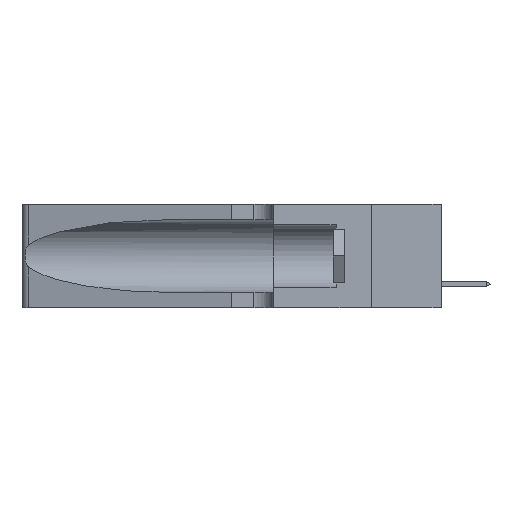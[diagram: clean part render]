
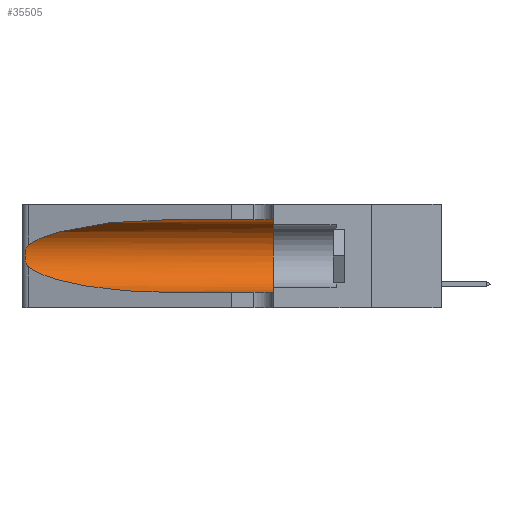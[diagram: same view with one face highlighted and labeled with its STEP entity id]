
A CAD part, left-side view. The second image highlights one B-rep face of the part: STEP entity #35505.
In plain terms, the highlighted cylindrical face has radius 3.308 mm (diameter 6.617 mm), a partial arc.
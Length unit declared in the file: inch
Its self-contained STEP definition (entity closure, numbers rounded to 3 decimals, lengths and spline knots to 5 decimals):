
#619 = CARTESIAN_POINT ( 'NONE',  ( 0.1305, 1.61858, 0.185 ) ) ;
#725 = DIRECTION ( 'NONE',  ( 0., -1., 0. ) ) ;
#741 = EDGE_CURVE ( 'NONE', #9641, #40267, #35137, .T. ) ;
#1351 = CARTESIAN_POINT ( 'NONE',  ( 0.25487, 1.22718, 0.14631 ) ) ;
#1749 = VERTEX_POINT ( 'NONE', #32545 ) ;
#2171 = CARTESIAN_POINT ( 'NONE',  ( 0.18966, 0.96281, 0.31525 ) ) ;
#2450 =( BOUNDED_CURVE ( )  B_SPLINE_CURVE ( 3, ( #1351, #26617, #44153, #33369 ),
 .UNSPECIFIED., .F., .T. ) 
 B_SPLINE_CURVE_WITH_KNOTS ( ( 4, 4 ),
 ( 3.44316, 4.71239 ),
 .UNSPECIFIED. ) 
 CURVE ( )  GEOMETRIC_REPRESENTATION_ITEM ( )  RATIONAL_B_SPLINE_CURVE ( ( 1., 0.87, 0.87, 1. ) ) 
 REPRESENTATION_ITEM ( '' )  );
#2625 = EDGE_CURVE ( 'NONE', #21936, #18528, #22553, .T. ) ;
#3529 = ORIENTED_EDGE ( 'NONE', *, *, #741, .T. ) ;
#3976 = CARTESIAN_POINT ( 'NONE',  ( 0.25787, 1.23484, 0.2124 ) ) ;
#4115 = DIRECTION ( 'NONE',  ( 0., 0., -1. ) ) ;
#6848 = EDGE_CURVE ( 'NONE', #1749, #18528, #18151, .T. ) ;
#7221 = CARTESIAN_POINT ( 'NONE',  ( 0.1305, 1.61858, 0.31525 ) ) ;
#7263 = LINE ( 'NONE', #7221, #25414 ) ;
#7407 = CARTESIAN_POINT ( 'NONE',  ( 0.26018, 1.23835, 0.19895 ) ) ;
#7546 = CARTESIAN_POINT ( 'NONE',  ( 0.26017, 1.23833, 0.17102 ) ) ;
#8415 = CARTESIAN_POINT ( 'NONE',  ( 0.1305, 0.72297, 0.05475 ) ) ;
#9257 = CARTESIAN_POINT ( 'NONE',  ( 0.25487, 1.22718, 0.22369 ) ) ;
#9641 = VERTEX_POINT ( 'NONE', #41501 ) ;
#10827 = CARTESIAN_POINT ( 'NONE',  ( 0.26075, 1.23896, 0.19203 ) ) ;
#10860 = DIRECTION ( 'NONE',  ( 0., 0., 1. ) ) ;
#12087 = VECTOR ( 'NONE', #15900, 39.37008 ) ;
#13704 = EDGE_LOOP ( 'NONE', ( #34426, #3529, #33341, #21244, #24357, #30673 ) ) ;
#14354 = CARTESIAN_POINT ( 'NONE',  ( 0.26075, 1.23896, 0.178 ) ) ;
#14659 = CARTESIAN_POINT ( 'NONE',  ( 0.25555, 1.22993, 0.14849 ) ) ;
#15741 = CARTESIAN_POINT ( 'NONE',  ( 0.1305, 1.61858, 0.05475 ) ) ;
#15900 = DIRECTION ( 'NONE',  ( 0., -1., 0. ) ) ;
#16974 = CARTESIAN_POINT ( 'NONE',  ( 0.25487, 1.22718, 0.14631 ) ) ;
#16994 = FACE_OUTER_BOUND ( 'NONE', #13704, .T. ) ;
#18151 = CIRCLE ( 'NONE', #33225, 0.13025 ) ;
#18528 = VERTEX_POINT ( 'NONE', #22972 ) ;
#21244 = ORIENTED_EDGE ( 'NONE', *, *, #2625, .T. ) ;
#21568 = CARTESIAN_POINT ( 'NONE',  ( 0.25639, 1.23184, 0.21858 ) ) ;
#21912 = EDGE_CURVE ( 'NONE', #40267, #21936, #2450, .T. ) ;
#21936 = VERTEX_POINT ( 'NONE', #8415 ) ;
#22180 = DIRECTION ( 'NONE',  ( 0., -1., 0. ) ) ;
#22553 = LINE ( 'NONE', #15741, #12087 ) ;
#22972 = CARTESIAN_POINT ( 'NONE',  ( 0.1305, 0.35, 0.05475 ) ) ;
#24114 = CYLINDRICAL_SURFACE ( 'NONE', #36951, 0.13025 ) ;
#24357 = ORIENTED_EDGE ( 'NONE', *, *, #6848, .F. ) ;
#25264 = CARTESIAN_POINT ( 'NONE',  ( 0.25487, 1.22718, 0.14631 ) ) ;
#25414 = VECTOR ( 'NONE', #725, 39.37008 ) ;
#26116 = CARTESIAN_POINT ( 'NONE',  ( 0.1305, 0.35, 0.185 ) ) ;
#26617 = CARTESIAN_POINT ( 'NONE',  ( 0.2373, 1.15595, 0.08982 ) ) ;
#28527 = CARTESIAN_POINT ( 'NONE',  ( 0.25555, 1.22994, 0.2215 ) ) ;
#29196 = DIRECTION ( 'NONE',  ( 0., 1., 0. ) ) ;
#30673 = ORIENTED_EDGE ( 'NONE', *, *, #34155, .F. ) ;
#30741 = CARTESIAN_POINT ( 'NONE',  ( 0.1305, 0.72297, 0.31525 ) ) ;
#32053 = CARTESIAN_POINT ( 'NONE',  ( 0.25789, 1.23486, 0.15765 ) ) ;
#32204 = CARTESIAN_POINT ( 'NONE',  ( 0.25854, 1.2359, 0.20912 ) ) ;
#32545 = CARTESIAN_POINT ( 'NONE',  ( 0.1305, 0.35, 0.31525 ) ) ;
#33225 = AXIS2_PLACEMENT_3D ( 'NONE', #26116, #29196, #10860 ) ;
#33341 = ORIENTED_EDGE ( 'NONE', *, *, #21912, .T. ) ;
#33369 = CARTESIAN_POINT ( 'NONE',  ( 0.1305, 0.72297, 0.05475 ) ) ;
#34155 = EDGE_CURVE ( 'NONE', #34254, #1749, #7263, .T. ) ;
#34158 = CARTESIAN_POINT ( 'NONE',  ( 0.2373, 1.15595, 0.28018 ) ) ;
#34254 = VERTEX_POINT ( 'NONE', #30741 ) ;
#34426 = ORIENTED_EDGE ( 'NONE', *, *, #40074, .T. ) ;
#35137 = B_SPLINE_CURVE_WITH_KNOTS ( 'NONE', 3,
 ( #42334, #28527, #21568, #3976, #32204, #7407, #10827, #14354, #7546, #38816, #32053, #35721, #14659, #25264 ),
 .UNSPECIFIED., .F., .F.,
 ( 4, 2, 2, 2, 2, 2, 4 ),
 ( 0., 0.00027, 0.00053, 0.00107, 0.0016, 0.00187, 0.00214 ),
 .UNSPECIFIED. ) ;
#35505 = ADVANCED_FACE ( 'NONE', ( #16994 ), #24114, .F. ) ;
#35721 = CARTESIAN_POINT ( 'NONE',  ( 0.25639, 1.23186, 0.15144 ) ) ;
#36951 = AXIS2_PLACEMENT_3D ( 'NONE', #619, #22180, #4115 ) ;
#38816 = CARTESIAN_POINT ( 'NONE',  ( 0.25856, 1.23593, 0.16098 ) ) ;
#40074 = EDGE_CURVE ( 'NONE', #34254, #9641, #44778, .T. ) ;
#40267 = VERTEX_POINT ( 'NONE', #16974 ) ;
#40790 = CARTESIAN_POINT ( 'NONE',  ( 0.1305, 0.72297, 0.31525 ) ) ;
#41501 = CARTESIAN_POINT ( 'NONE',  ( 0.25487, 1.22718, 0.22369 ) ) ;
#42334 = CARTESIAN_POINT ( 'NONE',  ( 0.25487, 1.22718, 0.22369 ) ) ;
#44153 = CARTESIAN_POINT ( 'NONE',  ( 0.18966, 0.96281, 0.05475 ) ) ;
#44778 =( BOUNDED_CURVE ( )  B_SPLINE_CURVE ( 3, ( #40790, #2171, #34158, #9257 ),
 .UNSPECIFIED., .F., .F. ) 
 B_SPLINE_CURVE_WITH_KNOTS ( ( 4, 4 ),
 ( 1.5708, 2.84003 ),
 .UNSPECIFIED. ) 
 CURVE ( )  GEOMETRIC_REPRESENTATION_ITEM ( )  RATIONAL_B_SPLINE_CURVE ( ( 1., 0.87, 0.87, 1. ) ) 
 REPRESENTATION_ITEM ( '' )  );
